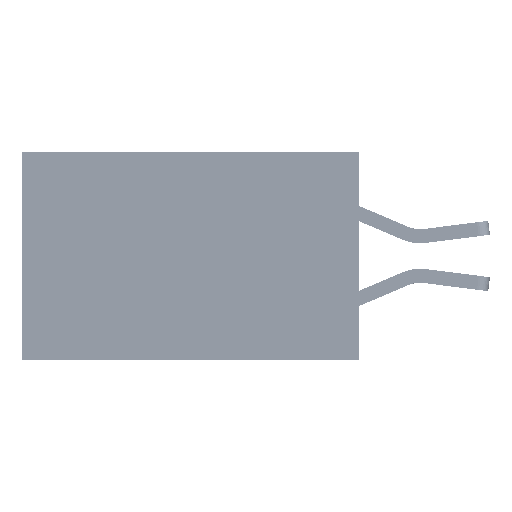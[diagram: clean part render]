
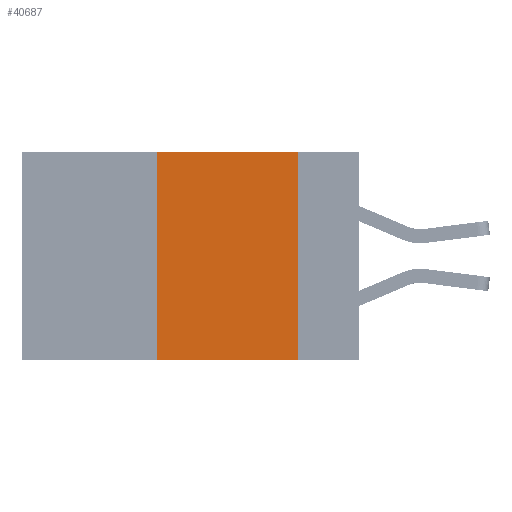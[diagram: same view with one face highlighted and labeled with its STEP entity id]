
A CAD part, left-side view. The second image highlights one B-rep face of the part: STEP entity #40687.
In plain terms, the highlighted planar face has unit normal (-1, 0, 0).
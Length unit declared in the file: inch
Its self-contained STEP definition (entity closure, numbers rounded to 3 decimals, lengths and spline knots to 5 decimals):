
#581 = ORIENTED_EDGE ( 'NONE', *, *, #28655, .F. ) ;
#775 = CARTESIAN_POINT ( 'NONE',  ( 0., 0.11, 0. ) ) ;
#2183 = VECTOR ( 'NONE', #8976, 39.37008 ) ;
#2398 = EDGE_CURVE ( 'NONE', #35336, #33755, #43541, .T. ) ;
#4678 = CARTESIAN_POINT ( 'NONE',  ( 0., 0.6, 0. ) ) ;
#4718 = FACE_OUTER_BOUND ( 'NONE', #32764, .T. ) ;
#6120 = ORIENTED_EDGE ( 'NONE', *, *, #38446, .T. ) ;
#7863 = DIRECTION ( 'NONE',  ( 0., 0., -1. ) ) ;
#7910 = PLANE ( 'NONE',  #9273 ) ;
#8061 = DIRECTION ( 'NONE',  ( 0., 0., -1. ) ) ;
#8976 = DIRECTION ( 'NONE',  ( 0., -1., 0. ) ) ;
#9045 = VECTOR ( 'NONE', #16515, 39.37008 ) ;
#9273 = AXIS2_PLACEMENT_3D ( 'NONE', #4678, #28670, #8061 ) ;
#9333 = VECTOR ( 'NONE', #7863, 39.37008 ) ;
#11818 = VECTOR ( 'NONE', #43219, 39.37008 ) ;
#14440 = CARTESIAN_POINT ( 'NONE',  ( 0., 0.36, -0.37 ) ) ;
#16515 = DIRECTION ( 'NONE',  ( 0., 0., 1. ) ) ;
#21971 = ORIENTED_EDGE ( 'NONE', *, *, #39170, .F. ) ;
#28450 = LINE ( 'NONE', #33033, #2183 ) ;
#28462 = CARTESIAN_POINT ( 'NONE',  ( 0., 0.11, 0. ) ) ;
#28655 = EDGE_CURVE ( 'NONE', #33297, #29874, #36818, .T. ) ;
#28670 = DIRECTION ( 'NONE',  ( 1., 0., 0. ) ) ;
#29874 = VERTEX_POINT ( 'NONE', #35609 ) ;
#30163 = LINE ( 'NONE', #39762, #11818 ) ;
#32764 = EDGE_LOOP ( 'NONE', ( #581, #21971, #43103, #6120 ) ) ;
#33033 = CARTESIAN_POINT ( 'NONE',  ( 0., 0.6, 0. ) ) ;
#33297 = VERTEX_POINT ( 'NONE', #775 ) ;
#33721 = CARTESIAN_POINT ( 'NONE',  ( 0., 0.36, 0. ) ) ;
#33755 = VERTEX_POINT ( 'NONE', #33871 ) ;
#33871 = CARTESIAN_POINT ( 'NONE',  ( 0., 0.36, 0. ) ) ;
#35336 = VERTEX_POINT ( 'NONE', #14440 ) ;
#35609 = CARTESIAN_POINT ( 'NONE',  ( 0., 0.11, -0.37 ) ) ;
#36818 = LINE ( 'NONE', #28462, #9333 ) ;
#38446 = EDGE_CURVE ( 'NONE', #35336, #29874, #30163, .T. ) ;
#39170 = EDGE_CURVE ( 'NONE', #33755, #33297, #28450, .T. ) ;
#39762 = CARTESIAN_POINT ( 'NONE',  ( 0., 0.6, -0.37 ) ) ;
#40687 = ADVANCED_FACE ( 'NONE', ( #4718 ), #7910, .F. ) ;
#43103 = ORIENTED_EDGE ( 'NONE', *, *, #2398, .F. ) ;
#43219 = DIRECTION ( 'NONE',  ( 0., -1., 0. ) ) ;
#43541 = LINE ( 'NONE', #33721, #9045 ) ;
